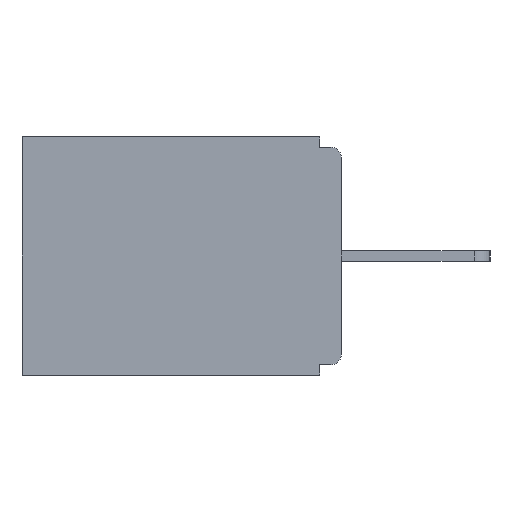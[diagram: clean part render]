
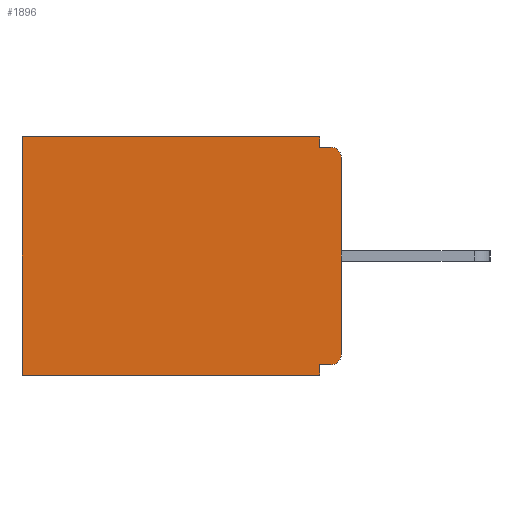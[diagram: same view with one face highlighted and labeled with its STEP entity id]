
A CAD part, left-side view. The second image highlights one B-rep face of the part: STEP entity #1896.
In plain terms, the highlighted planar face has unit normal (-1, 0, 0).
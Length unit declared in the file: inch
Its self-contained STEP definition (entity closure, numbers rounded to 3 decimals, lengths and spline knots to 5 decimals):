
#61 = DIRECTION ( 'NONE',  ( 0., 0., -1. ) ) ;
#978 = VECTOR ( 'NONE', #6470, 39.37008 ) ;
#1160 = EDGE_CURVE ( 'NONE', #6986, #14231, #2170, .T. ) ;
#1311 = LINE ( 'NONE', #2163, #8962 ) ;
#1399 = ORIENTED_EDGE ( 'NONE', *, *, #1160, .T. ) ;
#1603 = ORIENTED_EDGE ( 'NONE', *, *, #14325, .T. ) ;
#1739 = CARTESIAN_POINT ( 'NONE',  ( 0.298, 0.031, -0.343 ) ) ;
#1741 = CARTESIAN_POINT ( 'NONE',  ( 0.298, 0., 0. ) ) ;
#1896 = ADVANCED_FACE ( 'NONE', ( #10283 ), #10578, .F. ) ;
#1986 = LINE ( 'NONE', #13375, #16965 ) ;
#2105 = ORIENTED_EDGE ( 'NONE', *, *, #7332, .F. ) ;
#2163 = CARTESIAN_POINT ( 'NONE',  ( 0.298, 0., -0.328 ) ) ;
#2170 = CIRCLE ( 'NONE', #5771, 0.015 ) ;
#2235 = CARTESIAN_POINT ( 'NONE',  ( 0.298, 0., -0.015 ) ) ;
#2803 = VERTEX_POINT ( 'NONE', #10568 ) ;
#3010 = EDGE_CURVE ( 'NONE', #3083, #14231, #7412, .T. ) ;
#3083 = VERTEX_POINT ( 'NONE', #16503 ) ;
#3351 = VECTOR ( 'NONE', #8698, 39.37008 ) ;
#3367 = DIRECTION ( 'NONE',  ( 0., 0., -1. ) ) ;
#3405 = CARTESIAN_POINT ( 'NONE',  ( 0.298, 0., -0.343 ) ) ;
#3446 = CARTESIAN_POINT ( 'NONE',  ( 0.298, 0., -0.03 ) ) ;
#3588 = CARTESIAN_POINT ( 'NONE',  ( 0.298, 0.015, -0.328 ) ) ;
#3715 = VERTEX_POINT ( 'NONE', #14177 ) ;
#3909 = DIRECTION ( 'NONE',  ( 0., 0., -1. ) ) ;
#4323 = EDGE_LOOP ( 'NONE', ( #1399, #13370, #16886, #1603, #13540, #2105, #6729, #11155, #11628, #18711 ) ) ;
#4440 = AXIS2_PLACEMENT_3D ( 'NONE', #4581, #14673, #6087 ) ;
#4579 = CARTESIAN_POINT ( 'NONE',  ( 0.298, 0.46, 0. ) ) ;
#4581 = CARTESIAN_POINT ( 'NONE',  ( 0.298, 0.015, -0.313 ) ) ;
#4594 = EDGE_CURVE ( 'NONE', #18701, #3083, #16893, .T. ) ;
#5325 = VERTEX_POINT ( 'NONE', #4579 ) ;
#5451 = CARTESIAN_POINT ( 'NONE',  ( 0.298, 0.031, -0.343 ) ) ;
#5761 = LINE ( 'NONE', #1739, #9210 ) ;
#5771 = AXIS2_PLACEMENT_3D ( 'NONE', #18443, #12173, #61 ) ;
#5827 = CARTESIAN_POINT ( 'NONE',  ( 0.298, 0., 0. ) ) ;
#6087 = DIRECTION ( 'NONE',  ( 0., 0., -1. ) ) ;
#6470 = DIRECTION ( 'NONE',  ( 0., 0., -1. ) ) ;
#6729 = ORIENTED_EDGE ( 'NONE', *, *, #18339, .F. ) ;
#6844 = VERTEX_POINT ( 'NONE', #3588 ) ;
#6920 = VECTOR ( 'NONE', #14332, 39.37008 ) ;
#6986 = VERTEX_POINT ( 'NONE', #3446 ) ;
#7229 = CARTESIAN_POINT ( 'NONE',  ( 0.298, 0.031, 0. ) ) ;
#7332 = EDGE_CURVE ( 'NONE', #15605, #2803, #15381, .T. ) ;
#7350 = VERTEX_POINT ( 'NONE', #7834 ) ;
#7412 = LINE ( 'NONE', #2235, #3351 ) ;
#7528 = AXIS2_PLACEMENT_3D ( 'NONE', #5827, #11130, #11395 ) ;
#7834 = CARTESIAN_POINT ( 'NONE',  ( 0.298, 0.031, -0.328 ) ) ;
#8338 = DIRECTION ( 'NONE',  ( 0., 1., 0. ) ) ;
#8349 = DIRECTION ( 'NONE',  ( 0., 1., 0. ) ) ;
#8698 = DIRECTION ( 'NONE',  ( 0., -1., 0. ) ) ;
#8962 = VECTOR ( 'NONE', #8338, 39.37008 ) ;
#9210 = VECTOR ( 'NONE', #3367, 39.37008 ) ;
#9551 = VECTOR ( 'NONE', #3909, 39.37008 ) ;
#9779 = EDGE_CURVE ( 'NONE', #5325, #2803, #1986, .T. ) ;
#10283 = FACE_OUTER_BOUND ( 'NONE', #4323, .T. ) ;
#10568 = CARTESIAN_POINT ( 'NONE',  ( 0.298, 0.46, -0.343 ) ) ;
#10578 = PLANE ( 'NONE',  #7528 ) ;
#10880 = EDGE_CURVE ( 'NONE', #6986, #3715, #16529, .T. ) ;
#11130 = DIRECTION ( 'NONE',  ( 1., 0., 0. ) ) ;
#11155 = ORIENTED_EDGE ( 'NONE', *, *, #18571, .F. ) ;
#11395 = DIRECTION ( 'NONE',  ( 0., 0., -1. ) ) ;
#11585 = CARTESIAN_POINT ( 'NONE',  ( 0.298, 0., 0. ) ) ;
#11628 = ORIENTED_EDGE ( 'NONE', *, *, #12909, .T. ) ;
#12073 = DIRECTION ( 'NONE',  ( 0., 0., -1. ) ) ;
#12173 = DIRECTION ( 'NONE',  ( -1., 0., 0. ) ) ;
#12909 = EDGE_CURVE ( 'NONE', #6844, #3715, #15180, .T. ) ;
#13370 = ORIENTED_EDGE ( 'NONE', *, *, #3010, .F. ) ;
#13375 = CARTESIAN_POINT ( 'NONE',  ( 0.298, 0.46, 0. ) ) ;
#13540 = ORIENTED_EDGE ( 'NONE', *, *, #9779, .T. ) ;
#14161 = CARTESIAN_POINT ( 'NONE',  ( 0.298, 0.015, -0.015 ) ) ;
#14177 = CARTESIAN_POINT ( 'NONE',  ( 0.298, 0., -0.313 ) ) ;
#14231 = VERTEX_POINT ( 'NONE', #14161 ) ;
#14325 = EDGE_CURVE ( 'NONE', #18701, #5325, #17822, .T. ) ;
#14332 = DIRECTION ( 'NONE',  ( 0., 1., 0. ) ) ;
#14673 = DIRECTION ( 'NONE',  ( -1., 0., 0. ) ) ;
#15180 = CIRCLE ( 'NONE', #4440, 0.015 ) ;
#15381 = LINE ( 'NONE', #3405, #18488 ) ;
#15605 = VERTEX_POINT ( 'NONE', #18037 ) ;
#16503 = CARTESIAN_POINT ( 'NONE',  ( 0.298, 0.031, -0.015 ) ) ;
#16529 = LINE ( 'NONE', #1741, #978 ) ;
#16886 = ORIENTED_EDGE ( 'NONE', *, *, #4594, .F. ) ;
#16893 = LINE ( 'NONE', #5451, #9551 ) ;
#16965 = VECTOR ( 'NONE', #12073, 39.37008 ) ;
#17822 = LINE ( 'NONE', #11585, #6920 ) ;
#18037 = CARTESIAN_POINT ( 'NONE',  ( 0.298, 0.031, -0.343 ) ) ;
#18339 = EDGE_CURVE ( 'NONE', #7350, #15605, #5761, .T. ) ;
#18443 = CARTESIAN_POINT ( 'NONE',  ( 0.298, 0.015, -0.03 ) ) ;
#18488 = VECTOR ( 'NONE', #8349, 39.37008 ) ;
#18571 = EDGE_CURVE ( 'NONE', #6844, #7350, #1311, .T. ) ;
#18701 = VERTEX_POINT ( 'NONE', #7229 ) ;
#18711 = ORIENTED_EDGE ( 'NONE', *, *, #10880, .F. ) ;
